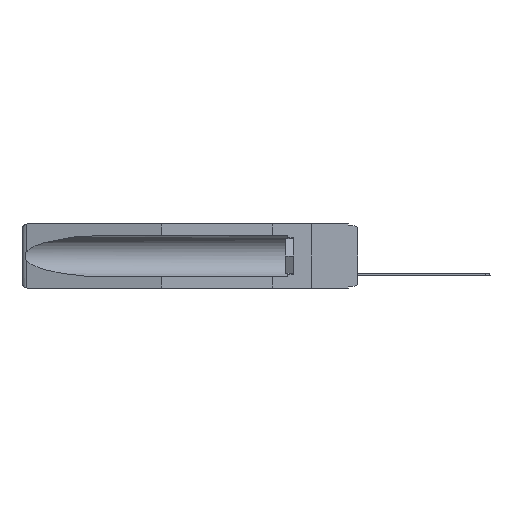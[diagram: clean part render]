
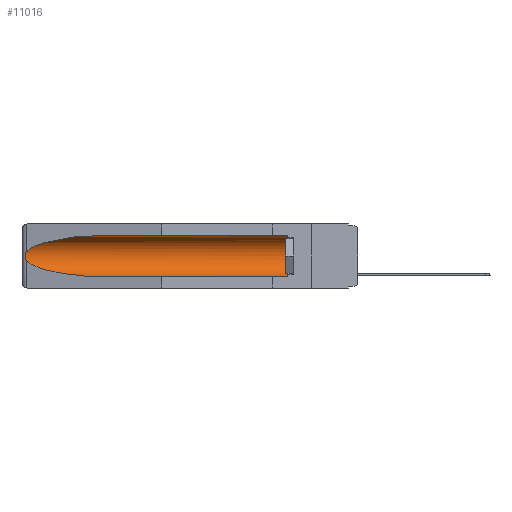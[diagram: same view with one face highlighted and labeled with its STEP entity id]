
A CAD part, left-side view. The second image highlights one B-rep face of the part: STEP entity #11016.
In plain terms, the highlighted cylindrical face has radius 2.857 mm (diameter 5.715 mm), a partial arc.
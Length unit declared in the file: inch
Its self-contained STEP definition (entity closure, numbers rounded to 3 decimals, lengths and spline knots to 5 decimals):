
#1084 = CARTESIAN_POINT ( 'NONE',  ( 0.26654, 1.53092, -0.15636 ) ) ;
#1173 = CARTESIAN_POINT ( 'NONE',  ( 0.26597, 1.52961, -0.15275 ) ) ;
#1404 = CARTESIAN_POINT ( 'NONE',  ( 0.26597, 1.5296, -0.19026 ) ) ;
#1476 = AXIS2_PLACEMENT_3D ( 'NONE', #5803, #2019, #17017 ) ;
#1517 = ORIENTED_EDGE ( 'NONE', *, *, #7596, .T. ) ;
#1523 = EDGE_CURVE ( 'NONE', #23870, #9229, #21822, .T. ) ;
#2019 = DIRECTION ( 'NONE',  ( 0., 1., 0. ) ) ;
#2884 = ORIENTED_EDGE ( 'NONE', *, *, #21370, .T. ) ;
#3271 = CARTESIAN_POINT ( 'NONE',  ( 0.155, -0.30754, -0.284 ) ) ;
#3373 = CYLINDRICAL_SURFACE ( 'NONE', #1476, 0.1125 ) ;
#4750 = DIRECTION ( 'NONE',  ( 0., -1., 0. ) ) ;
#4819 = CARTESIAN_POINT ( 'NONE',  ( 0.2675, 1.53308, -0.16763 ) ) ;
#5803 = CARTESIAN_POINT ( 'NONE',  ( 0.155, -0.30754, -0.1715 ) ) ;
#7051 = VECTOR ( 'NONE', #11083, 39.37008 ) ;
#7596 = EDGE_CURVE ( 'NONE', #9229, #17898, #17076, .T. ) ;
#8046 =( BOUNDED_CURVE ( )  B_SPLINE_CURVE ( 3, ( #15173, #11336, #9676, #15099 ),
 .UNSPECIFIED., .F., .F. ) 
 B_SPLINE_CURVE_WITH_KNOTS ( ( 4, 4 ),
 ( 0.1948, 1.5708 ),
 .UNSPECIFIED. ) 
 CURVE ( )  GEOMETRIC_REPRESENTATION_ITEM ( )  RATIONAL_B_SPLINE_CURVE ( ( 1., 0.848, 0.848, 1. ) ) 
 REPRESENTATION_ITEM ( '' )  );
#8410 = FACE_OUTER_BOUND ( 'NONE', #22911, .T. ) ;
#9097 = CARTESIAN_POINT ( 'NONE',  ( 0.21114, 1.30732, -0.059 ) ) ;
#9229 = VERTEX_POINT ( 'NONE', #17726 ) ;
#9676 = CARTESIAN_POINT ( 'NONE',  ( 0.21114, 1.30732, -0.284 ) ) ;
#10028 = ORIENTED_EDGE ( 'NONE', *, *, #21128, .T. ) ;
#10517 = CARTESIAN_POINT ( 'NONE',  ( 0.26655, 1.53094, -0.18657 ) ) ;
#10653 = DIRECTION ( 'NONE',  ( 0., 1., 0. ) ) ;
#10762 = CARTESIAN_POINT ( 'NONE',  ( 0.26537, 1.52718, -0.14972 ) ) ;
#11016 = ADVANCED_FACE ( 'NONE', ( #8410 ), #3373, .F. ) ;
#11083 = DIRECTION ( 'NONE',  ( 0., 1., 0. ) ) ;
#11336 = CARTESIAN_POINT ( 'NONE',  ( 0.25451, 1.48313, -0.24835 ) ) ;
#11406 = CARTESIAN_POINT ( 'NONE',  ( 0.155, 1.07973, -0.284 ) ) ;
#11474 = CARTESIAN_POINT ( 'NONE',  ( 0.26537, 1.52718, -0.14972 ) ) ;
#11537 =( BOUNDED_CURVE ( )  B_SPLINE_CURVE ( 3, ( #18220, #9097, #18401, #10762 ),
 .UNSPECIFIED., .F., .F. ) 
 B_SPLINE_CURVE_WITH_KNOTS ( ( 4, 4 ),
 ( 4.71239, 6.08839 ),
 .UNSPECIFIED. ) 
 CURVE ( )  GEOMETRIC_REPRESENTATION_ITEM ( )  RATIONAL_B_SPLINE_CURVE ( ( 1., 0.848, 0.848, 1. ) ) 
 REPRESENTATION_ITEM ( '' )  );
#11859 = VERTEX_POINT ( 'NONE', #11406 ) ;
#12263 = CARTESIAN_POINT ( 'NONE',  ( 0.155, 0.126, -0.1715 ) ) ;
#12787 = VERTEX_POINT ( 'NONE', #11474 ) ;
#13805 = EDGE_CURVE ( 'NONE', #17898, #12787, #11537, .T. ) ;
#13902 = CARTESIAN_POINT ( 'NONE',  ( 0.155, 0.126, -0.284 ) ) ;
#14445 = CARTESIAN_POINT ( 'NONE',  ( 0.26537, 1.52718, -0.14972 ) ) ;
#14829 = CARTESIAN_POINT ( 'NONE',  ( 0.155, -0.30754, -0.059 ) ) ;
#15099 = CARTESIAN_POINT ( 'NONE',  ( 0.155, 1.07973, -0.284 ) ) ;
#15173 = CARTESIAN_POINT ( 'NONE',  ( 0.26537, 1.52718, -0.19328 ) ) ;
#15604 = VERTEX_POINT ( 'NONE', #18179 ) ;
#15912 = AXIS2_PLACEMENT_3D ( 'NONE', #12263, #4750, #21918 ) ;
#17017 = DIRECTION ( 'NONE',  ( 0., 0., 1. ) ) ;
#17076 = LINE ( 'NONE', #14829, #7051 ) ;
#17603 = ORIENTED_EDGE ( 'NONE', *, *, #23469, .F. ) ;
#17726 = CARTESIAN_POINT ( 'NONE',  ( 0.155, 0.126, -0.059 ) ) ;
#17898 = VERTEX_POINT ( 'NONE', #19491 ) ;
#17996 = CARTESIAN_POINT ( 'NONE',  ( 0.26537, 1.52718, -0.19328 ) ) ;
#18076 = CARTESIAN_POINT ( 'NONE',  ( 0.2675, 1.53308, -0.17534 ) ) ;
#18179 = CARTESIAN_POINT ( 'NONE',  ( 0.26537, 1.52718, -0.19328 ) ) ;
#18220 = CARTESIAN_POINT ( 'NONE',  ( 0.155, 1.07973, -0.059 ) ) ;
#18401 = CARTESIAN_POINT ( 'NONE',  ( 0.25451, 1.48313, -0.09465 ) ) ;
#18755 = VECTOR ( 'NONE', #10653, 39.37008 ) ;
#18924 = B_SPLINE_CURVE_WITH_KNOTS ( 'NONE', 3,
 ( #14445, #1173, #1084, #23978, #4819, #18076, #21827, #10517, #1404, #17996 ),
 .UNSPECIFIED., .F., .F.,
 ( 4, 2, 2, 2, 4 ),
 ( 0., 0.00029, 0.00058, 0.00087, 0.00117 ),
 .UNSPECIFIED. ) ;
#19491 = CARTESIAN_POINT ( 'NONE',  ( 0.155, 1.07973, -0.059 ) ) ;
#21128 = EDGE_CURVE ( 'NONE', #12787, #15604, #18924, .T. ) ;
#21354 = ORIENTED_EDGE ( 'NONE', *, *, #1523, .T. ) ;
#21370 = EDGE_CURVE ( 'NONE', #15604, #11859, #8046, .T. ) ;
#21822 = CIRCLE ( 'NONE', #15912, 0.1125 ) ;
#21827 = CARTESIAN_POINT ( 'NONE',  ( 0.2673, 1.53269, -0.17917 ) ) ;
#21918 = DIRECTION ( 'NONE',  ( 0., 0., 1. ) ) ;
#22440 = ORIENTED_EDGE ( 'NONE', *, *, #13805, .T. ) ;
#22911 = EDGE_LOOP ( 'NONE', ( #22440, #10028, #2884, #17603, #21354, #1517 ) ) ;
#23469 = EDGE_CURVE ( 'NONE', #23870, #11859, #24408, .T. ) ;
#23870 = VERTEX_POINT ( 'NONE', #13902 ) ;
#23978 = CARTESIAN_POINT ( 'NONE',  ( 0.2673, 1.5327, -0.16383 ) ) ;
#24408 = LINE ( 'NONE', #3271, #18755 ) ;
